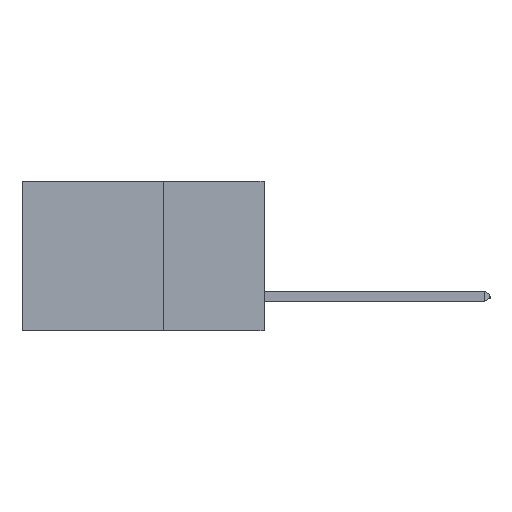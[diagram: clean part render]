
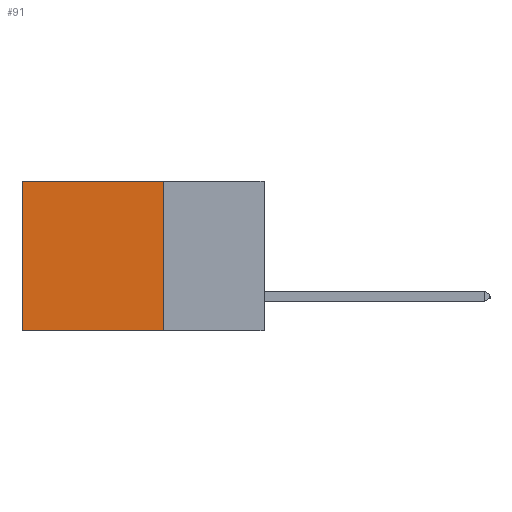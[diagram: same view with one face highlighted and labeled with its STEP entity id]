
A CAD part, left-side view. The second image highlights one B-rep face of the part: STEP entity #91.
In plain terms, the highlighted planar face has unit normal (-1, 0, 0).
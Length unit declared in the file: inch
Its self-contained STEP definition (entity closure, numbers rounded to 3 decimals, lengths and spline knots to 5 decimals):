
#91 = ADVANCED_FACE ( 'NONE', ( #4205 ), #12315, .F. ) ;
#269 = CARTESIAN_POINT ( 'NONE',  ( 0.298, 0.6, 0. ) ) ;
#1157 = VERTEX_POINT ( 'NONE', #12346 ) ;
#1182 = LINE ( 'NONE', #8050, #6321 ) ;
#2798 = EDGE_CURVE ( 'NONE', #1157, #11346, #1182, .T. ) ;
#3015 = EDGE_LOOP ( 'NONE', ( #6440, #10536, #11247, #8393 ) ) ;
#3161 = VERTEX_POINT ( 'NONE', #10323 ) ;
#3910 = CARTESIAN_POINT ( 'NONE',  ( 0.298, 0.6, 0. ) ) ;
#4205 = FACE_OUTER_BOUND ( 'NONE', #3015, .T. ) ;
#4450 = VECTOR ( 'NONE', #8478, 39.37008 ) ;
#5440 = LINE ( 'NONE', #10178, #10250 ) ;
#5954 = LINE ( 'NONE', #7228, #10726 ) ;
#6035 = CARTESIAN_POINT ( 'NONE',  ( 0.298, 0.25, -0.37 ) ) ;
#6321 = VECTOR ( 'NONE', #7056, 39.37008 ) ;
#6440 = ORIENTED_EDGE ( 'NONE', *, *, #8276, .T. ) ;
#6747 = DIRECTION ( 'NONE',  ( 1., 0., 0. ) ) ;
#7031 = DIRECTION ( 'NONE',  ( 0., 0., -1. ) ) ;
#7056 = DIRECTION ( 'NONE',  ( 0., 1., 0. ) ) ;
#7142 = LINE ( 'NONE', #269, #4450 ) ;
#7228 = CARTESIAN_POINT ( 'NONE',  ( 0.298, 0.25, -0.37 ) ) ;
#7338 = VERTEX_POINT ( 'NONE', #6035 ) ;
#8050 = CARTESIAN_POINT ( 'NONE',  ( 0.298, 0.25, 0. ) ) ;
#8276 = EDGE_CURVE ( 'NONE', #11346, #3161, #7142, .T. ) ;
#8393 = ORIENTED_EDGE ( 'NONE', *, *, #2798, .T. ) ;
#8478 = DIRECTION ( 'NONE',  ( 0., 0., -1. ) ) ;
#9043 = AXIS2_PLACEMENT_3D ( 'NONE', #12526, #6747, #7031 ) ;
#10048 = DIRECTION ( 'NONE',  ( 0., 1., 0. ) ) ;
#10178 = CARTESIAN_POINT ( 'NONE',  ( 0.298, 0.25, 0. ) ) ;
#10250 = VECTOR ( 'NONE', #11077, 39.37008 ) ;
#10323 = CARTESIAN_POINT ( 'NONE',  ( 0.298, 0.6, -0.37 ) ) ;
#10477 = EDGE_CURVE ( 'NONE', #7338, #3161, #5954, .T. ) ;
#10536 = ORIENTED_EDGE ( 'NONE', *, *, #10477, .F. ) ;
#10726 = VECTOR ( 'NONE', #10048, 39.37008 ) ;
#11077 = DIRECTION ( 'NONE',  ( 0., 0., -1. ) ) ;
#11247 = ORIENTED_EDGE ( 'NONE', *, *, #11908, .F. ) ;
#11346 = VERTEX_POINT ( 'NONE', #3910 ) ;
#11908 = EDGE_CURVE ( 'NONE', #1157, #7338, #5440, .T. ) ;
#12315 = PLANE ( 'NONE',  #9043 ) ;
#12346 = CARTESIAN_POINT ( 'NONE',  ( 0.298, 0.25, 0. ) ) ;
#12526 = CARTESIAN_POINT ( 'NONE',  ( 0.298, 0.25, 0. ) ) ;
